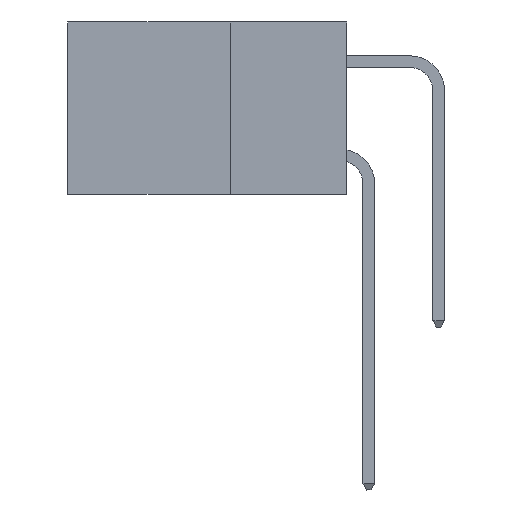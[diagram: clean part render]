
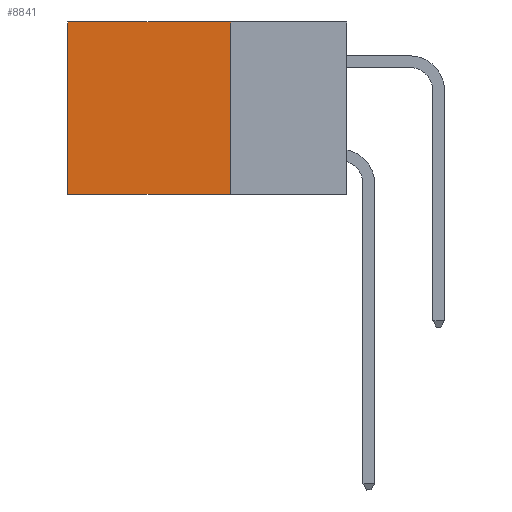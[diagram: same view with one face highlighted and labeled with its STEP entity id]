
A CAD part, left-side view. The second image highlights one B-rep face of the part: STEP entity #8841.
In plain terms, the highlighted planar face has unit normal (-1, 0, 0).
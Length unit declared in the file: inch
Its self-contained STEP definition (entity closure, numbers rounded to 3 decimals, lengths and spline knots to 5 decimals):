
#64 = VECTOR ( 'NONE', #7511, 39.37008 ) ;
#397 = LINE ( 'NONE', #5047, #64 ) ;
#764 = VERTEX_POINT ( 'NONE', #12082 ) ;
#1295 = LINE ( 'NONE', #3816, #7507 ) ;
#1437 = LINE ( 'NONE', #2848, #13783 ) ;
#2848 = CARTESIAN_POINT ( 'NONE',  ( 0.2875, 0.25, 0. ) ) ;
#3072 = DIRECTION ( 'NONE',  ( 1., 0., 0. ) ) ;
#3228 = VERTEX_POINT ( 'NONE', #3973 ) ;
#3727 = ORIENTED_EDGE ( 'NONE', *, *, #4783, .T. ) ;
#3816 = CARTESIAN_POINT ( 'NONE',  ( 0.2875, 0.6, 0. ) ) ;
#3866 = DIRECTION ( 'NONE',  ( 0., 0., -1. ) ) ;
#3973 = CARTESIAN_POINT ( 'NONE',  ( 0.2875, 0.25, 0. ) ) ;
#4183 = LINE ( 'NONE', #12398, #12729 ) ;
#4783 = EDGE_CURVE ( 'NONE', #764, #13695, #1295, .T. ) ;
#5047 = CARTESIAN_POINT ( 'NONE',  ( 0.2875, 0.25, 0. ) ) ;
#5346 = EDGE_LOOP ( 'NONE', ( #3727, #6325, #7043, #7856 ) ) ;
#5694 = DIRECTION ( 'NONE',  ( 0., 1., 0. ) ) ;
#5698 = EDGE_CURVE ( 'NONE', #3228, #11158, #397, .T. ) ;
#6325 = ORIENTED_EDGE ( 'NONE', *, *, #7973, .F. ) ;
#6431 = DIRECTION ( 'NONE',  ( 0., 0., -1. ) ) ;
#7043 = ORIENTED_EDGE ( 'NONE', *, *, #5698, .F. ) ;
#7507 = VECTOR ( 'NONE', #3866, 39.37008 ) ;
#7511 = DIRECTION ( 'NONE',  ( 0., 0., -1. ) ) ;
#7682 = CARTESIAN_POINT ( 'NONE',  ( 0.2875, 0.25, 0. ) ) ;
#7856 = ORIENTED_EDGE ( 'NONE', *, *, #12170, .T. ) ;
#7973 = EDGE_CURVE ( 'NONE', #11158, #13695, #4183, .T. ) ;
#8555 = CARTESIAN_POINT ( 'NONE',  ( 0.2875, 0.25, -0.37 ) ) ;
#8841 = ADVANCED_FACE ( 'NONE', ( #9990 ), #13217, .F. ) ;
#9990 = FACE_OUTER_BOUND ( 'NONE', #5346, .T. ) ;
#10986 = CARTESIAN_POINT ( 'NONE',  ( 0.2875, 0.6, -0.37 ) ) ;
#11158 = VERTEX_POINT ( 'NONE', #8555 ) ;
#11773 = DIRECTION ( 'NONE',  ( 0., 1., 0. ) ) ;
#12082 = CARTESIAN_POINT ( 'NONE',  ( 0.2875, 0.6, 0. ) ) ;
#12170 = EDGE_CURVE ( 'NONE', #3228, #764, #1437, .T. ) ;
#12398 = CARTESIAN_POINT ( 'NONE',  ( 0.2875, 0.25, -0.37 ) ) ;
#12729 = VECTOR ( 'NONE', #5694, 39.37008 ) ;
#12744 = AXIS2_PLACEMENT_3D ( 'NONE', #7682, #3072, #6431 ) ;
#13217 = PLANE ( 'NONE',  #12744 ) ;
#13695 = VERTEX_POINT ( 'NONE', #10986 ) ;
#13783 = VECTOR ( 'NONE', #11773, 39.37008 ) ;
